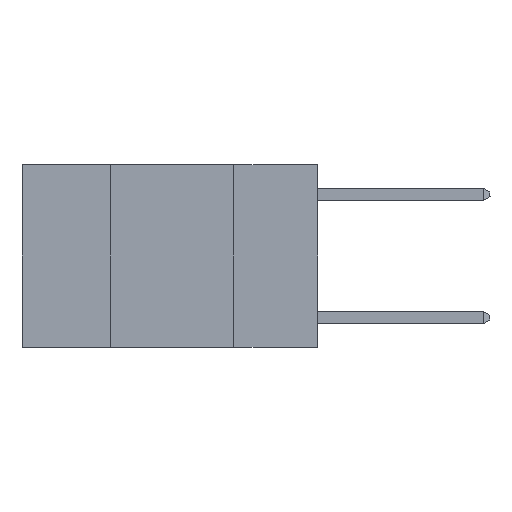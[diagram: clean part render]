
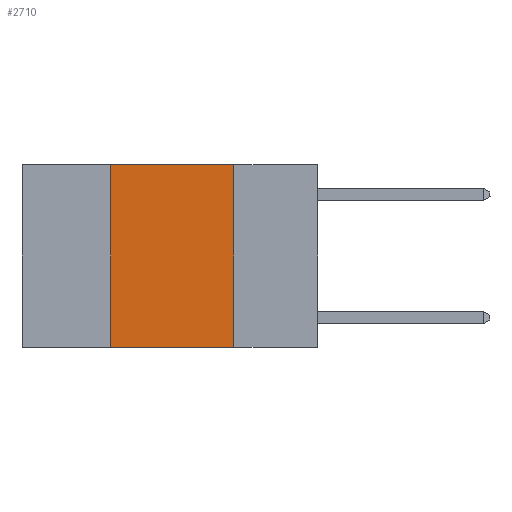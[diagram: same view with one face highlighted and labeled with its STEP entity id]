
A CAD part, left-side view. The second image highlights one B-rep face of the part: STEP entity #2710.
In plain terms, the highlighted planar face has unit normal (-1, 0, 0).
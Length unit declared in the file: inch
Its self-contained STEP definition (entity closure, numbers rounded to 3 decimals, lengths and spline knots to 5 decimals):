
#454 = EDGE_CURVE ( 'NONE', #8806, #7108, #2802, .T. ) ;
#1313 = EDGE_LOOP ( 'NONE', ( #3817, #4051, #4179, #5398 ) ) ;
#1604 = LINE ( 'NONE', #14660, #14729 ) ;
#1606 = CARTESIAN_POINT ( 'NONE',  ( 0., 0.17, 0. ) ) ;
#1804 = VECTOR ( 'NONE', #13871, 39.37008 ) ;
#1815 = VECTOR ( 'NONE', #10636, 39.37008 ) ;
#2414 = DIRECTION ( 'NONE',  ( 0., 0., -1. ) ) ;
#2710 = ADVANCED_FACE ( 'NONE', ( #14345 ), #11273, .F. ) ;
#2802 = LINE ( 'NONE', #7541, #15758 ) ;
#3817 = ORIENTED_EDGE ( 'NONE', *, *, #9174, .F. ) ;
#4051 = ORIENTED_EDGE ( 'NONE', *, *, #10597, .F. ) ;
#4179 = ORIENTED_EDGE ( 'NONE', *, *, #454, .F. ) ;
#5398 = ORIENTED_EDGE ( 'NONE', *, *, #9472, .T. ) ;
#6454 = CARTESIAN_POINT ( 'NONE',  ( 0., 0.6, 0. ) ) ;
#7108 = VERTEX_POINT ( 'NONE', #11546 ) ;
#7541 = CARTESIAN_POINT ( 'NONE',  ( 0., 0.42, 0. ) ) ;
#8150 = AXIS2_PLACEMENT_3D ( 'NONE', #6454, #10153, #2414 ) ;
#8740 = DIRECTION ( 'NONE',  ( 0., 0., 1. ) ) ;
#8752 = VERTEX_POINT ( 'NONE', #11311 ) ;
#8806 = VERTEX_POINT ( 'NONE', #11361 ) ;
#8946 = VERTEX_POINT ( 'NONE', #11512 ) ;
#9174 = EDGE_CURVE ( 'NONE', #8752, #8946, #11983, .T. ) ;
#9472 = EDGE_CURVE ( 'NONE', #8806, #8946, #1604, .T. ) ;
#10153 = DIRECTION ( 'NONE',  ( 1., 0., 0. ) ) ;
#10597 = EDGE_CURVE ( 'NONE', #7108, #8752, #11969, .T. ) ;
#10636 = DIRECTION ( 'NONE',  ( 0., 0., -1. ) ) ;
#11273 = PLANE ( 'NONE',  #8150 ) ;
#11311 = CARTESIAN_POINT ( 'NONE',  ( 0., 0.17, 0. ) ) ;
#11361 = CARTESIAN_POINT ( 'NONE',  ( 0., 0.42, -0.37 ) ) ;
#11512 = CARTESIAN_POINT ( 'NONE',  ( 0., 0.17, -0.37 ) ) ;
#11546 = CARTESIAN_POINT ( 'NONE',  ( 0., 0.42, 0. ) ) ;
#11969 = LINE ( 'NONE', #12611, #1804 ) ;
#11983 = LINE ( 'NONE', #1606, #1815 ) ;
#12611 = CARTESIAN_POINT ( 'NONE',  ( 0., 0.6, 0. ) ) ;
#13455 = DIRECTION ( 'NONE',  ( 0., -1., 0. ) ) ;
#13871 = DIRECTION ( 'NONE',  ( 0., -1., 0. ) ) ;
#14345 = FACE_OUTER_BOUND ( 'NONE', #1313, .T. ) ;
#14660 = CARTESIAN_POINT ( 'NONE',  ( 0., 0.6, -0.37 ) ) ;
#14729 = VECTOR ( 'NONE', #13455, 39.37008 ) ;
#15758 = VECTOR ( 'NONE', #8740, 39.37008 ) ;
